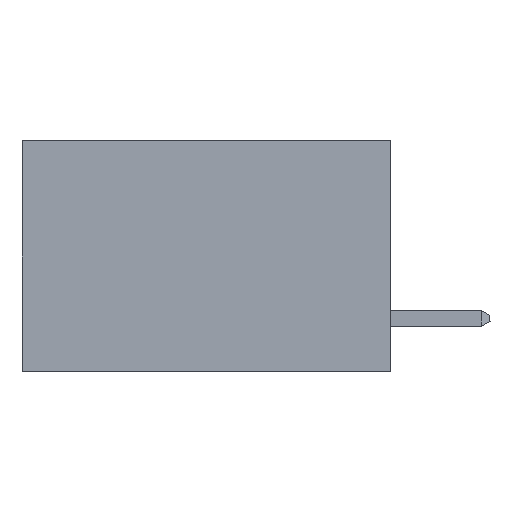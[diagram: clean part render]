
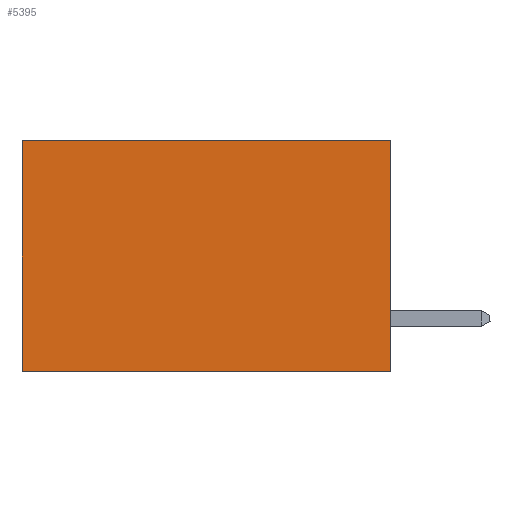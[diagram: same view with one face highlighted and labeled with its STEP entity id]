
A CAD part, left-side view. The second image highlights one B-rep face of the part: STEP entity #5395.
In plain terms, the highlighted planar face has unit normal (-1, 0, 0).
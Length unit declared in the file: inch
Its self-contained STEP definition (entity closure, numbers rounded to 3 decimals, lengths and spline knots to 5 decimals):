
#548 = ORIENTED_EDGE ( 'NONE', *, *, #11646, .T. ) ;
#759 = CARTESIAN_POINT ( 'NONE',  ( 0.277, 0.59, -0.37 ) ) ;
#867 = VECTOR ( 'NONE', #8352, 39.37008 ) ;
#1427 = CARTESIAN_POINT ( 'NONE',  ( 0.277, 0., 0. ) ) ;
#1476 = VERTEX_POINT ( 'NONE', #12743 ) ;
#1701 = EDGE_CURVE ( 'NONE', #11907, #17938, #6622, .T. ) ;
#2104 = VECTOR ( 'NONE', #3785, 39.37008 ) ;
#3302 = VERTEX_POINT ( 'NONE', #7923 ) ;
#3785 = DIRECTION ( 'NONE',  ( 0., 1., 0. ) ) ;
#4311 = AXIS2_PLACEMENT_3D ( 'NONE', #14010, #13944, #13855 ) ;
#5395 = ADVANCED_FACE ( 'NONE', ( #14173 ), #14528, .F. ) ;
#5460 = EDGE_CURVE ( 'NONE', #11907, #3302, #17741, .T. ) ;
#6526 = CARTESIAN_POINT ( 'NONE',  ( 0.277, 0., -0.37 ) ) ;
#6622 = LINE ( 'NONE', #15623, #15011 ) ;
#7923 = CARTESIAN_POINT ( 'NONE',  ( 0.277, 0.59, 0. ) ) ;
#8063 = ORIENTED_EDGE ( 'NONE', *, *, #1701, .F. ) ;
#8261 = CARTESIAN_POINT ( 'NONE',  ( 0.277, 0., -0.37 ) ) ;
#8352 = DIRECTION ( 'NONE',  ( 0., 0., -1. ) ) ;
#8825 = EDGE_LOOP ( 'NONE', ( #548, #18478, #8063, #18252 ) ) ;
#11260 = DIRECTION ( 'NONE',  ( 0., 1., 0. ) ) ;
#11622 = CARTESIAN_POINT ( 'NONE',  ( 0.277, 0., 0. ) ) ;
#11646 = EDGE_CURVE ( 'NONE', #3302, #1476, #12826, .T. ) ;
#11907 = VERTEX_POINT ( 'NONE', #1427 ) ;
#12743 = CARTESIAN_POINT ( 'NONE',  ( 0.277, 0.59, -0.37 ) ) ;
#12826 = LINE ( 'NONE', #759, #867 ) ;
#13855 = DIRECTION ( 'NONE',  ( 0., 0., -1. ) ) ;
#13944 = DIRECTION ( 'NONE',  ( 1., 0., 0. ) ) ;
#14010 = CARTESIAN_POINT ( 'NONE',  ( 0.277, 0., -0.37 ) ) ;
#14173 = FACE_OUTER_BOUND ( 'NONE', #8825, .T. ) ;
#14528 = PLANE ( 'NONE',  #4311 ) ;
#15011 = VECTOR ( 'NONE', #16194, 39.37008 ) ;
#15623 = CARTESIAN_POINT ( 'NONE',  ( 0.277, 0., -0.37 ) ) ;
#16146 = EDGE_CURVE ( 'NONE', #17938, #1476, #18073, .T. ) ;
#16194 = DIRECTION ( 'NONE',  ( 0., 0., -1. ) ) ;
#16799 = VECTOR ( 'NONE', #11260, 39.37008 ) ;
#17741 = LINE ( 'NONE', #11622, #16799 ) ;
#17938 = VERTEX_POINT ( 'NONE', #6526 ) ;
#18073 = LINE ( 'NONE', #8261, #2104 ) ;
#18252 = ORIENTED_EDGE ( 'NONE', *, *, #5460, .T. ) ;
#18478 = ORIENTED_EDGE ( 'NONE', *, *, #16146, .F. ) ;
